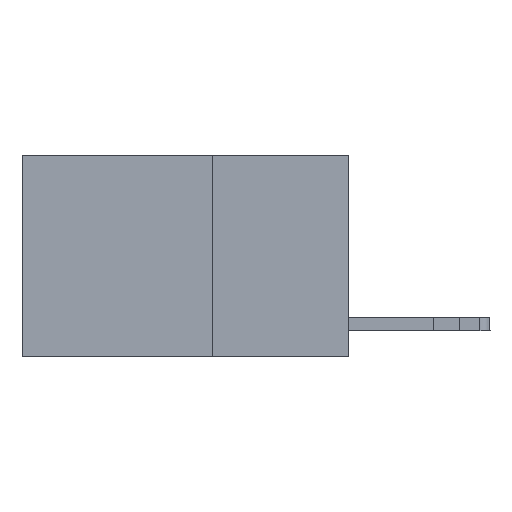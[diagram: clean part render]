
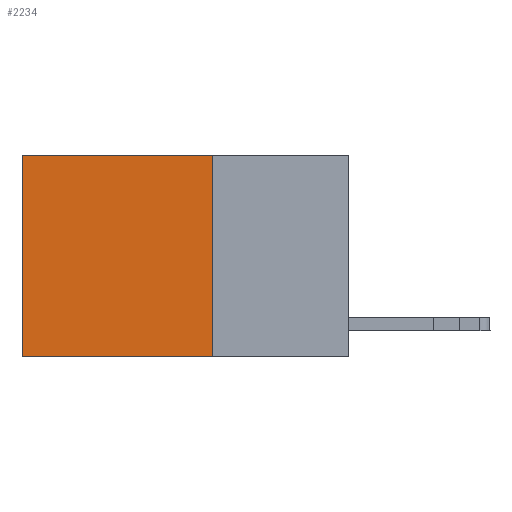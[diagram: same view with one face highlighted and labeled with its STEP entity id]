
A CAD part, left-side view. The second image highlights one B-rep face of the part: STEP entity #2234.
In plain terms, the highlighted planar face has unit normal (-1, 0, 0).
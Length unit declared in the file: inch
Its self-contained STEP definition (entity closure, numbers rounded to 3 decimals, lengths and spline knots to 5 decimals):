
#165 = CARTESIAN_POINT ( 'NONE',  ( 0.2625, 0.25, 0. ) ) ;
#396 = LINE ( 'NONE', #2090, #7052 ) ;
#475 = CARTESIAN_POINT ( 'NONE',  ( 0.2625, 0.6, 0. ) ) ;
#902 = ORIENTED_EDGE ( 'NONE', *, *, #1475, .T. ) ;
#1089 = DIRECTION ( 'NONE',  ( 1., 0., 0. ) ) ;
#1144 = DIRECTION ( 'NONE',  ( 0., 0., -1. ) ) ;
#1170 = EDGE_CURVE ( 'NONE', #1718, #11828, #11615, .T. ) ;
#1475 = EDGE_CURVE ( 'NONE', #2082, #11828, #396, .T. ) ;
#1666 = VERTEX_POINT ( 'NONE', #5451 ) ;
#1718 = VERTEX_POINT ( 'NONE', #6352 ) ;
#2082 = VERTEX_POINT ( 'NONE', #475 ) ;
#2090 = CARTESIAN_POINT ( 'NONE',  ( 0.2625, 0.6, 0. ) ) ;
#2234 = ADVANCED_FACE ( 'NONE', ( #5660 ), #8393, .F. ) ;
#3491 = CARTESIAN_POINT ( 'NONE',  ( 0.2625, 0.6, -0.37 ) ) ;
#3960 = AXIS2_PLACEMENT_3D ( 'NONE', #165, #1089, #1144 ) ;
#4070 = DIRECTION ( 'NONE',  ( 0., 0., -1. ) ) ;
#4277 = VECTOR ( 'NONE', #5103, 39.37008 ) ;
#4311 = LINE ( 'NONE', #6941, #4277 ) ;
#4512 = CARTESIAN_POINT ( 'NONE',  ( 0.2625, 0.25, -0.37 ) ) ;
#5103 = DIRECTION ( 'NONE',  ( 0., 1., 0. ) ) ;
#5316 = ORIENTED_EDGE ( 'NONE', *, *, #1170, .F. ) ;
#5451 = CARTESIAN_POINT ( 'NONE',  ( 0.2625, 0.25, 0. ) ) ;
#5660 = FACE_OUTER_BOUND ( 'NONE', #10442, .T. ) ;
#6352 = CARTESIAN_POINT ( 'NONE',  ( 0.2625, 0.25, -0.37 ) ) ;
#6824 = EDGE_CURVE ( 'NONE', #1666, #2082, #4311, .T. ) ;
#6941 = CARTESIAN_POINT ( 'NONE',  ( 0.2625, 0.25, 0. ) ) ;
#7052 = VECTOR ( 'NONE', #4070, 39.37008 ) ;
#7083 = DIRECTION ( 'NONE',  ( 0., 1., 0. ) ) ;
#8201 = ORIENTED_EDGE ( 'NONE', *, *, #10828, .F. ) ;
#8286 = CARTESIAN_POINT ( 'NONE',  ( 0.2625, 0.25, 0. ) ) ;
#8393 = PLANE ( 'NONE',  #3960 ) ;
#9954 = LINE ( 'NONE', #8286, #11738 ) ;
#10442 = EDGE_LOOP ( 'NONE', ( #902, #5316, #8201, #11451 ) ) ;
#10828 = EDGE_CURVE ( 'NONE', #1666, #1718, #9954, .T. ) ;
#11141 = DIRECTION ( 'NONE',  ( 0., 0., -1. ) ) ;
#11451 = ORIENTED_EDGE ( 'NONE', *, *, #6824, .T. ) ;
#11615 = LINE ( 'NONE', #4512, #11650 ) ;
#11650 = VECTOR ( 'NONE', #7083, 39.37008 ) ;
#11738 = VECTOR ( 'NONE', #11141, 39.37008 ) ;
#11828 = VERTEX_POINT ( 'NONE', #3491 ) ;
